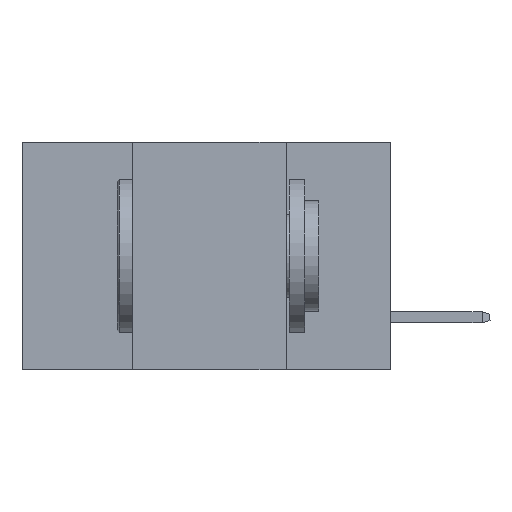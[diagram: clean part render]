
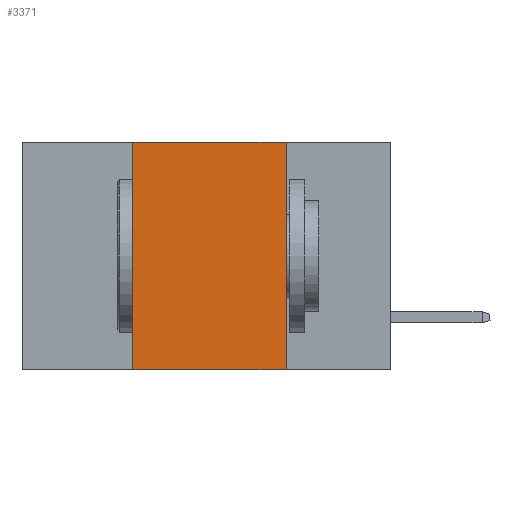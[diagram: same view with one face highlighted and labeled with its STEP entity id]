
A CAD part, left-side view. The second image highlights one B-rep face of the part: STEP entity #3371.
In plain terms, the highlighted planar face has unit normal (-1, 0, 0).
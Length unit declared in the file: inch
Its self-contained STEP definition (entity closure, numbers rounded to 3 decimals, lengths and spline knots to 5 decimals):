
#119 = VERTEX_POINT ( 'NONE', #11286 ) ;
#621 = EDGE_CURVE ( 'NONE', #119, #8770, #716, .T. ) ;
#716 = LINE ( 'NONE', #6153, #5549 ) ;
#1670 = VERTEX_POINT ( 'NONE', #11106 ) ;
#1715 = LINE ( 'NONE', #3773, #3995 ) ;
#1954 = AXIS2_PLACEMENT_3D ( 'NONE', #6073, #6033, #5955 ) ;
#2771 = VERTEX_POINT ( 'NONE', #10397 ) ;
#3371 = ADVANCED_FACE ( 'NONE', ( #3494 ), #6157, .F. ) ;
#3494 = FACE_OUTER_BOUND ( 'NONE', #8410, .T. ) ;
#3773 = CARTESIAN_POINT ( 'NONE',  ( 0., 0.6, -0.37 ) ) ;
#3995 = VECTOR ( 'NONE', #11088, 39.37008 ) ;
#4359 = EDGE_CURVE ( 'NONE', #1670, #119, #7263, .T. ) ;
#5549 = VECTOR ( 'NONE', #6182, 39.37008 ) ;
#5955 = DIRECTION ( 'NONE',  ( 0., 0., -1. ) ) ;
#5960 = CARTESIAN_POINT ( 'NONE',  ( 0., 0.42, 0. ) ) ;
#6033 = DIRECTION ( 'NONE',  ( 1., 0., 0. ) ) ;
#6037 = LINE ( 'NONE', #5960, #10598 ) ;
#6073 = CARTESIAN_POINT ( 'NONE',  ( 0., 0.6, 0. ) ) ;
#6153 = CARTESIAN_POINT ( 'NONE',  ( 0., 0.17, 0. ) ) ;
#6157 = PLANE ( 'NONE',  #1954 ) ;
#6182 = DIRECTION ( 'NONE',  ( 0., 0., -1. ) ) ;
#6938 = EDGE_CURVE ( 'NONE', #2771, #8770, #1715, .T. ) ;
#7215 = EDGE_CURVE ( 'NONE', #2771, #1670, #6037, .T. ) ;
#7263 = LINE ( 'NONE', #7574, #12015 ) ;
#7574 = CARTESIAN_POINT ( 'NONE',  ( 0., 0.6, 0. ) ) ;
#8410 = EDGE_LOOP ( 'NONE', ( #8825, #10639, #9603, #9648 ) ) ;
#8425 = DIRECTION ( 'NONE',  ( 0., -1., 0. ) ) ;
#8770 = VERTEX_POINT ( 'NONE', #10193 ) ;
#8825 = ORIENTED_EDGE ( 'NONE', *, *, #621, .F. ) ;
#9603 = ORIENTED_EDGE ( 'NONE', *, *, #7215, .F. ) ;
#9648 = ORIENTED_EDGE ( 'NONE', *, *, #6938, .T. ) ;
#10193 = CARTESIAN_POINT ( 'NONE',  ( 0., 0.17, -0.37 ) ) ;
#10397 = CARTESIAN_POINT ( 'NONE',  ( 0., 0.42, -0.37 ) ) ;
#10598 = VECTOR ( 'NONE', #11405, 39.37008 ) ;
#10639 = ORIENTED_EDGE ( 'NONE', *, *, #4359, .F. ) ;
#11088 = DIRECTION ( 'NONE',  ( 0., -1., 0. ) ) ;
#11106 = CARTESIAN_POINT ( 'NONE',  ( 0., 0.42, 0. ) ) ;
#11286 = CARTESIAN_POINT ( 'NONE',  ( 0., 0.17, 0. ) ) ;
#11405 = DIRECTION ( 'NONE',  ( 0., 0., 1. ) ) ;
#12015 = VECTOR ( 'NONE', #8425, 39.37008 ) ;
